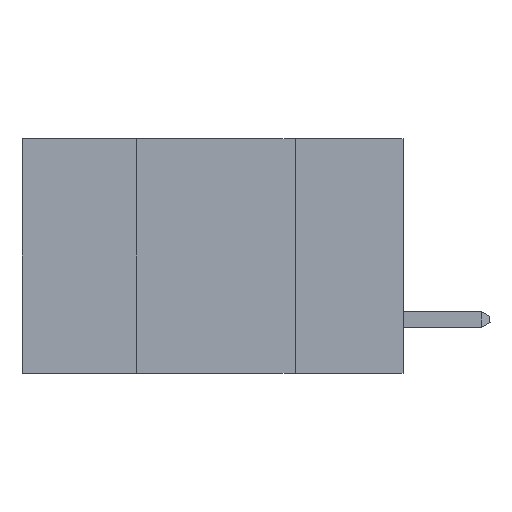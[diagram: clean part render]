
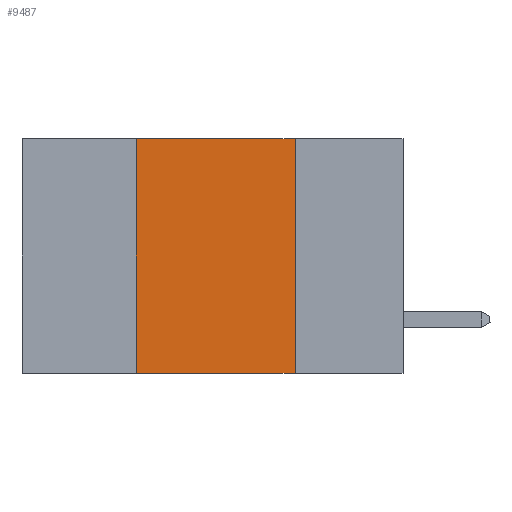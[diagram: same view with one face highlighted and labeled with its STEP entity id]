
A CAD part, left-side view. The second image highlights one B-rep face of the part: STEP entity #9487.
In plain terms, the highlighted planar face has unit normal (-1, 0, 0).
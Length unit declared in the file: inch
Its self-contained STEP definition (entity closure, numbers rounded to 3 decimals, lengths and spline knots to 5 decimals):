
#70 = CARTESIAN_POINT ( 'NONE',  ( 0., 0.6, 0. ) ) ;
#80 = CARTESIAN_POINT ( 'NONE',  ( 0., 0.42, 0. ) ) ;
#226 = DIRECTION ( 'NONE',  ( 0., -1., 0. ) ) ;
#1805 = CARTESIAN_POINT ( 'NONE',  ( 0., 0.42, -0.37 ) ) ;
#2616 = ORIENTED_EDGE ( 'NONE', *, *, #5220, .F. ) ;
#2766 = LINE ( 'NONE', #80, #5671 ) ;
#2856 = EDGE_CURVE ( 'NONE', #6278, #11604, #10787, .T. ) ;
#3098 = CARTESIAN_POINT ( 'NONE',  ( 0., 0.6, -0.37 ) ) ;
#3858 = CARTESIAN_POINT ( 'NONE',  ( 0., 0.42, 0. ) ) ;
#3895 = DIRECTION ( 'NONE',  ( 0., 0., 1. ) ) ;
#4041 = DIRECTION ( 'NONE',  ( 0., -1., 0. ) ) ;
#4119 = EDGE_CURVE ( 'NONE', #6140, #4843, #9566, .T. ) ;
#4631 = ORIENTED_EDGE ( 'NONE', *, *, #11932, .F. ) ;
#4705 = VECTOR ( 'NONE', #4041, 39.37008 ) ;
#4843 = VERTEX_POINT ( 'NONE', #11249 ) ;
#5220 = EDGE_CURVE ( 'NONE', #6140, #6278, #2766, .T. ) ;
#5255 = CARTESIAN_POINT ( 'NONE',  ( 0., 0.17, 0. ) ) ;
#5671 = VECTOR ( 'NONE', #3895, 39.37008 ) ;
#6140 = VERTEX_POINT ( 'NONE', #1805 ) ;
#6278 = VERTEX_POINT ( 'NONE', #3858 ) ;
#6350 = FACE_OUTER_BOUND ( 'NONE', #7121, .T. ) ;
#6478 = DIRECTION ( 'NONE',  ( 1., 0., 0. ) ) ;
#6521 = CARTESIAN_POINT ( 'NONE',  ( 0., 0.6, 0. ) ) ;
#7103 = DIRECTION ( 'NONE',  ( 0., 0., -1. ) ) ;
#7121 = EDGE_LOOP ( 'NONE', ( #4631, #9523, #2616, #8929 ) ) ;
#7292 = DIRECTION ( 'NONE',  ( 0., 0., -1. ) ) ;
#7877 = CARTESIAN_POINT ( 'NONE',  ( 0., 0.17, 0. ) ) ;
#8291 = VECTOR ( 'NONE', #226, 39.37008 ) ;
#8541 = VECTOR ( 'NONE', #7103, 39.37008 ) ;
#8929 = ORIENTED_EDGE ( 'NONE', *, *, #4119, .T. ) ;
#9001 = AXIS2_PLACEMENT_3D ( 'NONE', #6521, #6478, #7292 ) ;
#9487 = ADVANCED_FACE ( 'NONE', ( #6350 ), #10179, .F. ) ;
#9523 = ORIENTED_EDGE ( 'NONE', *, *, #2856, .F. ) ;
#9566 = LINE ( 'NONE', #3098, #4705 ) ;
#10179 = PLANE ( 'NONE',  #9001 ) ;
#10787 = LINE ( 'NONE', #70, #8291 ) ;
#10901 = LINE ( 'NONE', #5255, #8541 ) ;
#11249 = CARTESIAN_POINT ( 'NONE',  ( 0., 0.17, -0.37 ) ) ;
#11604 = VERTEX_POINT ( 'NONE', #7877 ) ;
#11932 = EDGE_CURVE ( 'NONE', #11604, #4843, #10901, .T. ) ;
